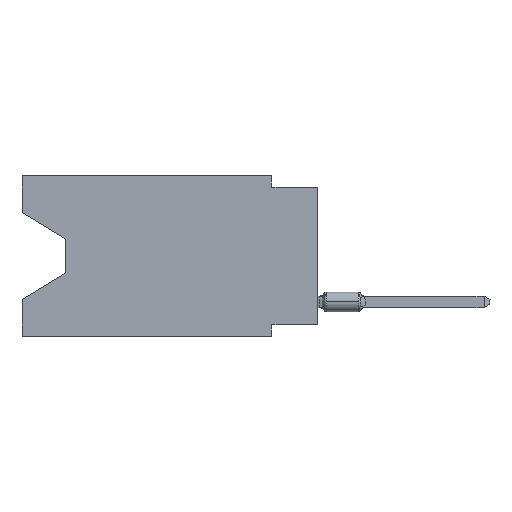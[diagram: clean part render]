
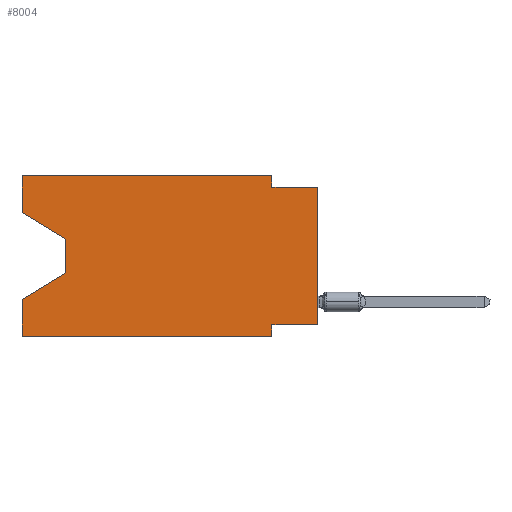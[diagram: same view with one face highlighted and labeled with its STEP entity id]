
A CAD part, left-side view. The second image highlights one B-rep face of the part: STEP entity #8004.
In plain terms, the highlighted planar face has unit normal (-1, 0, 0).
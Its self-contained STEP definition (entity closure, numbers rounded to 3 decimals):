
#45 = ORIENTED_EDGE ( 'NONE', *, *, #11224, .F. ) ;
#162 = ORIENTED_EDGE ( 'NONE', *, *, #8603, .F. ) ;
#299 = CARTESIAN_POINT ( 'NONE',  ( 0., 16.383, -6.852 ) ) ;
#308 = VERTEX_POINT ( 'NONE', #12435 ) ;
#759 = VECTOR ( 'NONE', #8539, 1000. ) ;
#936 = CARTESIAN_POINT ( 'NONE',  ( 0., 16.383, 0. ) ) ;
#1410 = CARTESIAN_POINT ( 'NONE',  ( 0., 16.383, -8.89 ) ) ;
#1486 = ORIENTED_EDGE ( 'NONE', *, *, #3010, .F. ) ;
#1917 = VERTEX_POINT ( 'NONE', #4923 ) ;
#1956 = LINE ( 'NONE', #12170, #2437 ) ;
#1987 = DIRECTION ( 'NONE',  ( 0., 0., -1. ) ) ;
#2028 = CARTESIAN_POINT ( 'NONE',  ( 0., 16.383, -8.89 ) ) ;
#2206 = LINE ( 'NONE', #7765, #6288 ) ;
#2285 = LINE ( 'NONE', #11442, #6914 ) ;
#2437 = VECTOR ( 'NONE', #8936, 1000. ) ;
#2459 = ORIENTED_EDGE ( 'NONE', *, *, #2896, .T. ) ;
#2855 = EDGE_CURVE ( 'NONE', #7581, #13927, #11080, .T. ) ;
#2877 = VECTOR ( 'NONE', #7819, 1000. ) ;
#2896 = EDGE_CURVE ( 'NONE', #7162, #6139, #3029, .T. ) ;
#3010 = EDGE_CURVE ( 'NONE', #11011, #6593, #9337, .T. ) ;
#3019 = ORIENTED_EDGE ( 'NONE', *, *, #11219, .T. ) ;
#3029 = LINE ( 'NONE', #3109, #3491 ) ;
#3109 = CARTESIAN_POINT ( 'NONE',  ( 0., 13.97, -3.505 ) ) ;
#3181 = DIRECTION ( 'NONE',  ( 0., -0.855, -0.519 ) ) ;
#3219 = CARTESIAN_POINT ( 'NONE',  ( 0., 2.54, 0. ) ) ;
#3334 = DIRECTION ( 'NONE',  ( 0., 0., -1. ) ) ;
#3491 = VECTOR ( 'NONE', #3334, 1000. ) ;
#3560 = VECTOR ( 'NONE', #7873, 1000. ) ;
#3653 = EDGE_CURVE ( 'NONE', #308, #5906, #1956, .T. ) ;
#4201 = VECTOR ( 'NONE', #11155, 1000. ) ;
#4315 = CARTESIAN_POINT ( 'NONE',  ( 0., 16.383, 0. ) ) ;
#4338 = LINE ( 'NONE', #2028, #3560 ) ;
#4901 = DIRECTION ( 'NONE',  ( 0., 0., 1. ) ) ;
#4923 = CARTESIAN_POINT ( 'NONE',  ( 0., 0., -8.255 ) ) ;
#5078 = CARTESIAN_POINT ( 'NONE',  ( 0., 0., 0. ) ) ;
#5177 = VERTEX_POINT ( 'NONE', #299 ) ;
#5811 = VECTOR ( 'NONE', #3181, 1000. ) ;
#5906 = VERTEX_POINT ( 'NONE', #10826 ) ;
#5929 = ORIENTED_EDGE ( 'NONE', *, *, #3653, .F. ) ;
#6139 = VERTEX_POINT ( 'NONE', #9744 ) ;
#6288 = VECTOR ( 'NONE', #1987, 1000. ) ;
#6509 = VERTEX_POINT ( 'NONE', #1410 ) ;
#6593 = VERTEX_POINT ( 'NONE', #13056 ) ;
#6855 = DIRECTION ( 'NONE',  ( 0., 0., 1. ) ) ;
#6914 = VECTOR ( 'NONE', #6855, 1000. ) ;
#7162 = VERTEX_POINT ( 'NONE', #12125 ) ;
#7483 = VECTOR ( 'NONE', #12255, 1000. ) ;
#7581 = VERTEX_POINT ( 'NONE', #14723 ) ;
#7709 = DIRECTION ( 'NONE',  ( 0., 0., -1. ) ) ;
#7749 = LINE ( 'NONE', #11275, #2877 ) ;
#7765 = CARTESIAN_POINT ( 'NONE',  ( 0., 2.54, 0. ) ) ;
#7819 = DIRECTION ( 'NONE',  ( 0., 1., 0. ) ) ;
#7873 = DIRECTION ( 'NONE',  ( 0., -1., 0. ) ) ;
#8004 = ADVANCED_FACE ( 'NONE', ( #14783 ), #12218, .F. ) ;
#8420 = VECTOR ( 'NONE', #9124, 1000. ) ;
#8442 = ORIENTED_EDGE ( 'NONE', *, *, #11785, .T. ) ;
#8539 = DIRECTION ( 'NONE',  ( 0., 0., 1. ) ) ;
#8603 = EDGE_CURVE ( 'NONE', #9162, #7581, #9264, .T. ) ;
#8723 = EDGE_CURVE ( 'NONE', #1917, #11011, #7749, .T. ) ;
#8936 = DIRECTION ( 'NONE',  ( 0., -1., 0. ) ) ;
#9124 = DIRECTION ( 'NONE',  ( 0., 0., -1. ) ) ;
#9162 = VERTEX_POINT ( 'NONE', #12392 ) ;
#9264 = LINE ( 'NONE', #10536, #10804 ) ;
#9337 = LINE ( 'NONE', #10322, #8420 ) ;
#9515 = LINE ( 'NONE', #5078, #759 ) ;
#9744 = CARTESIAN_POINT ( 'NONE',  ( 0., 13.97, -5.385 ) ) ;
#10066 = LINE ( 'NONE', #10766, #7483 ) ;
#10088 = CARTESIAN_POINT ( 'NONE',  ( 0., 16.383, -2.038 ) ) ;
#10311 = LINE ( 'NONE', #10088, #5811 ) ;
#10322 = CARTESIAN_POINT ( 'NONE',  ( 0., 2.54, -8.89 ) ) ;
#10529 = ORIENTED_EDGE ( 'NONE', *, *, #12563, .F. ) ;
#10536 = CARTESIAN_POINT ( 'NONE',  ( 0., 16.383, 0. ) ) ;
#10766 = CARTESIAN_POINT ( 'NONE',  ( 0., 13.97, -5.385 ) ) ;
#10804 = VECTOR ( 'NONE', #4901, 1000. ) ;
#10826 = CARTESIAN_POINT ( 'NONE',  ( 0., 0., -0.635 ) ) ;
#11011 = VERTEX_POINT ( 'NONE', #12822 ) ;
#11080 = LINE ( 'NONE', #936, #4201 ) ;
#11155 = DIRECTION ( 'NONE',  ( 0., -1., 0. ) ) ;
#11219 = EDGE_CURVE ( 'NONE', #9162, #7162, #10311, .T. ) ;
#11224 = EDGE_CURVE ( 'NONE', #13927, #308, #2206, .T. ) ;
#11275 = CARTESIAN_POINT ( 'NONE',  ( 0., 0., -8.255 ) ) ;
#11386 = DIRECTION ( 'NONE',  ( 1., 0., 0. ) ) ;
#11442 = CARTESIAN_POINT ( 'NONE',  ( 0., 16.383, 0. ) ) ;
#11605 = ORIENTED_EDGE ( 'NONE', *, *, #13290, .T. ) ;
#11785 = EDGE_CURVE ( 'NONE', #1917, #5906, #9515, .T. ) ;
#12030 = ORIENTED_EDGE ( 'NONE', *, *, #8723, .F. ) ;
#12125 = CARTESIAN_POINT ( 'NONE',  ( 0., 13.97, -3.505 ) ) ;
#12170 = CARTESIAN_POINT ( 'NONE',  ( 0., 0., -0.635 ) ) ;
#12218 = PLANE ( 'NONE',  #13668 ) ;
#12255 = DIRECTION ( 'NONE',  ( 0., 0.855, -0.519 ) ) ;
#12392 = CARTESIAN_POINT ( 'NONE',  ( 0., 16.383, -2.038 ) ) ;
#12435 = CARTESIAN_POINT ( 'NONE',  ( 0., 2.54, -0.635 ) ) ;
#12563 = EDGE_CURVE ( 'NONE', #6509, #5177, #2285, .T. ) ;
#12822 = CARTESIAN_POINT ( 'NONE',  ( 0., 2.54, -8.255 ) ) ;
#12869 = ORIENTED_EDGE ( 'NONE', *, *, #2855, .F. ) ;
#13056 = CARTESIAN_POINT ( 'NONE',  ( 0., 2.54, -8.89 ) ) ;
#13290 = EDGE_CURVE ( 'NONE', #6509, #6593, #4338, .T. ) ;
#13562 = EDGE_LOOP ( 'NONE', ( #3019, #2459, #13972, #10529, #11605, #1486, #12030, #8442, #5929, #45, #12869, #162 ) ) ;
#13668 = AXIS2_PLACEMENT_3D ( 'NONE', #4315, #11386, #7709 ) ;
#13859 = EDGE_CURVE ( 'NONE', #6139, #5177, #10066, .T. ) ;
#13927 = VERTEX_POINT ( 'NONE', #3219 ) ;
#13972 = ORIENTED_EDGE ( 'NONE', *, *, #13859, .T. ) ;
#14723 = CARTESIAN_POINT ( 'NONE',  ( 0., 16.383, 0. ) ) ;
#14783 = FACE_OUTER_BOUND ( 'NONE', #13562, .T. ) ;
